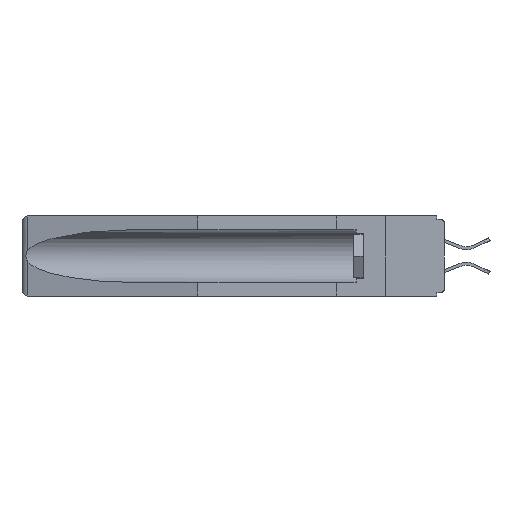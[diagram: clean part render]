
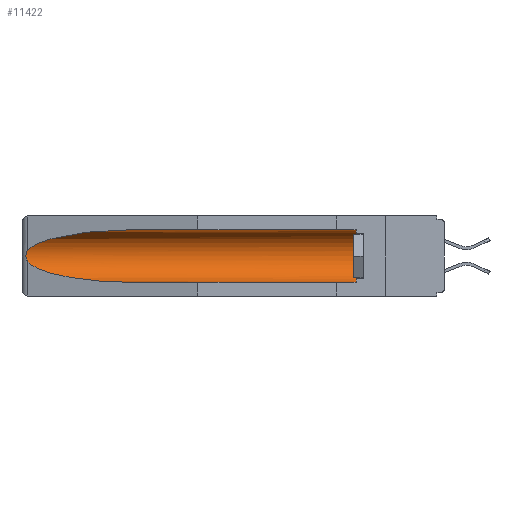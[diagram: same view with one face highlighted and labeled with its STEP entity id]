
A CAD part, left-side view. The second image highlights one B-rep face of the part: STEP entity #11422.
In plain terms, the highlighted cylindrical face has radius 2.857 mm (diameter 5.715 mm), a partial arc.
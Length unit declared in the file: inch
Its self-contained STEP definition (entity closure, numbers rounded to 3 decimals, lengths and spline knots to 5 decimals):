
#85 = AXIS2_PLACEMENT_3D ( 'NONE', #12126, #13989, #3013 ) ;
#228 = CARTESIAN_POINT ( 'NONE',  ( 0.155, 1.07973, -0.059 ) ) ;
#586 = CARTESIAN_POINT ( 'NONE',  ( 0.155, 0.126, -0.284 ) ) ;
#910 = EDGE_CURVE ( 'NONE', #18032, #17523, #10907, .T. ) ;
#994 = CARTESIAN_POINT ( 'NONE',  ( 0.155, 0.126, -0.1715 ) ) ;
#2720 =( BOUNDED_CURVE ( )  B_SPLINE_CURVE ( 3, ( #20797, #15249, #18666, #22478 ),
 .UNSPECIFIED., .F., .F. ) 
 B_SPLINE_CURVE_WITH_KNOTS ( ( 4, 4 ),
 ( 4.71239, 6.08839 ),
 .UNSPECIFIED. ) 
 CURVE ( )  GEOMETRIC_REPRESENTATION_ITEM ( )  RATIONAL_B_SPLINE_CURVE ( ( 1., 0.848, 0.848, 1. ) ) 
 REPRESENTATION_ITEM ( '' )  );
#3013 = DIRECTION ( 'NONE',  ( 0., 0., 1. ) ) ;
#3239 = CARTESIAN_POINT ( 'NONE',  ( 0.2675, 1.53308, -0.17534 ) ) ;
#3554 = CARTESIAN_POINT ( 'NONE',  ( 0.2673, 1.5327, -0.16383 ) ) ;
#4030 = ORIENTED_EDGE ( 'NONE', *, *, #12783, .T. ) ;
#4340 = CYLINDRICAL_SURFACE ( 'NONE', #85, 0.1125 ) ;
#5230 = DIRECTION ( 'NONE',  ( 0., 1., 0. ) ) ;
#5262 = CARTESIAN_POINT ( 'NONE',  ( 0.2673, 1.53269, -0.17917 ) ) ;
#5462 = CARTESIAN_POINT ( 'NONE',  ( 0.155, 1.07973, -0.284 ) ) ;
#5736 = VERTEX_POINT ( 'NONE', #228 ) ;
#6182 = ORIENTED_EDGE ( 'NONE', *, *, #910, .F. ) ;
#6947 = CARTESIAN_POINT ( 'NONE',  ( 0.155, 1.07973, -0.284 ) ) ;
#7276 = CARTESIAN_POINT ( 'NONE',  ( 0.26537, 1.52718, -0.19328 ) ) ;
#8036 = DIRECTION ( 'NONE',  ( 0., -1., 0. ) ) ;
#8272 = ORIENTED_EDGE ( 'NONE', *, *, #21123, .T. ) ;
#8609 = B_SPLINE_CURVE_WITH_KNOTS ( 'NONE', 3,
 ( #17671, #15769, #17839, #3554, #21487, #3239, #5262, #15682, #21405, #12215 ),
 .UNSPECIFIED., .F., .F.,
 ( 4, 2, 2, 2, 4 ),
 ( 0., 0.00029, 0.00058, 0.00087, 0.00117 ),
 .UNSPECIFIED. ) ;
#8957 = DIRECTION ( 'NONE',  ( 0., 1., 0. ) ) ;
#10273 = EDGE_CURVE ( 'NONE', #12994, #5736, #16383, .T. ) ;
#10464 = CARTESIAN_POINT ( 'NONE',  ( 0.25451, 1.48313, -0.24835 ) ) ;
#10582 = AXIS2_PLACEMENT_3D ( 'NONE', #994, #8036, #15195 ) ;
#10907 = LINE ( 'NONE', #12448, #11192 ) ;
#11192 = VECTOR ( 'NONE', #8957, 39.37008 ) ;
#11422 = ADVANCED_FACE ( 'NONE', ( #17729 ), #4340, .F. ) ;
#12126 = CARTESIAN_POINT ( 'NONE',  ( 0.155, -0.30754, -0.1715 ) ) ;
#12215 = CARTESIAN_POINT ( 'NONE',  ( 0.26537, 1.52718, -0.19328 ) ) ;
#12448 = CARTESIAN_POINT ( 'NONE',  ( 0.155, -0.30754, -0.284 ) ) ;
#12457 = EDGE_LOOP ( 'NONE', ( #12914, #8272, #15364, #6182, #4030, #15777 ) ) ;
#12762 =( BOUNDED_CURVE ( )  B_SPLINE_CURVE ( 3, ( #19235, #10464, #17431, #6947 ),
 .UNSPECIFIED., .F., .F. ) 
 B_SPLINE_CURVE_WITH_KNOTS ( ( 4, 4 ),
 ( 0.1948, 1.5708 ),
 .UNSPECIFIED. ) 
 CURVE ( )  GEOMETRIC_REPRESENTATION_ITEM ( )  RATIONAL_B_SPLINE_CURVE ( ( 1., 0.848, 0.848, 1. ) ) 
 REPRESENTATION_ITEM ( '' )  );
#12783 = EDGE_CURVE ( 'NONE', #18032, #12994, #19670, .T. ) ;
#12914 = ORIENTED_EDGE ( 'NONE', *, *, #13014, .T. ) ;
#12994 = VERTEX_POINT ( 'NONE', #13218 ) ;
#13014 = EDGE_CURVE ( 'NONE', #5736, #22300, #2720, .T. ) ;
#13218 = CARTESIAN_POINT ( 'NONE',  ( 0.155, 0.126, -0.059 ) ) ;
#13251 = VERTEX_POINT ( 'NONE', #7276 ) ;
#13989 = DIRECTION ( 'NONE',  ( 0., 1., 0. ) ) ;
#15195 = DIRECTION ( 'NONE',  ( 0., 0., 1. ) ) ;
#15249 = CARTESIAN_POINT ( 'NONE',  ( 0.21114, 1.30732, -0.059 ) ) ;
#15364 = ORIENTED_EDGE ( 'NONE', *, *, #17923, .T. ) ;
#15682 = CARTESIAN_POINT ( 'NONE',  ( 0.26655, 1.53094, -0.18657 ) ) ;
#15769 = CARTESIAN_POINT ( 'NONE',  ( 0.26597, 1.52961, -0.15275 ) ) ;
#15777 = ORIENTED_EDGE ( 'NONE', *, *, #10273, .T. ) ;
#16383 = LINE ( 'NONE', #19872, #18886 ) ;
#17431 = CARTESIAN_POINT ( 'NONE',  ( 0.21114, 1.30732, -0.284 ) ) ;
#17523 = VERTEX_POINT ( 'NONE', #5462 ) ;
#17671 = CARTESIAN_POINT ( 'NONE',  ( 0.26537, 1.52718, -0.14972 ) ) ;
#17729 = FACE_OUTER_BOUND ( 'NONE', #12457, .T. ) ;
#17839 = CARTESIAN_POINT ( 'NONE',  ( 0.26654, 1.53092, -0.15636 ) ) ;
#17923 = EDGE_CURVE ( 'NONE', #13251, #17523, #12762, .T. ) ;
#18032 = VERTEX_POINT ( 'NONE', #586 ) ;
#18666 = CARTESIAN_POINT ( 'NONE',  ( 0.25451, 1.48313, -0.09465 ) ) ;
#18886 = VECTOR ( 'NONE', #5230, 39.37008 ) ;
#19235 = CARTESIAN_POINT ( 'NONE',  ( 0.26537, 1.52718, -0.19328 ) ) ;
#19670 = CIRCLE ( 'NONE', #10582, 0.1125 ) ;
#19872 = CARTESIAN_POINT ( 'NONE',  ( 0.155, -0.30754, -0.059 ) ) ;
#20797 = CARTESIAN_POINT ( 'NONE',  ( 0.155, 1.07973, -0.059 ) ) ;
#21065 = CARTESIAN_POINT ( 'NONE',  ( 0.26537, 1.52718, -0.14972 ) ) ;
#21123 = EDGE_CURVE ( 'NONE', #22300, #13251, #8609, .T. ) ;
#21405 = CARTESIAN_POINT ( 'NONE',  ( 0.26597, 1.5296, -0.19026 ) ) ;
#21487 = CARTESIAN_POINT ( 'NONE',  ( 0.2675, 1.53308, -0.16763 ) ) ;
#22300 = VERTEX_POINT ( 'NONE', #21065 ) ;
#22478 = CARTESIAN_POINT ( 'NONE',  ( 0.26537, 1.52718, -0.14972 ) ) ;
